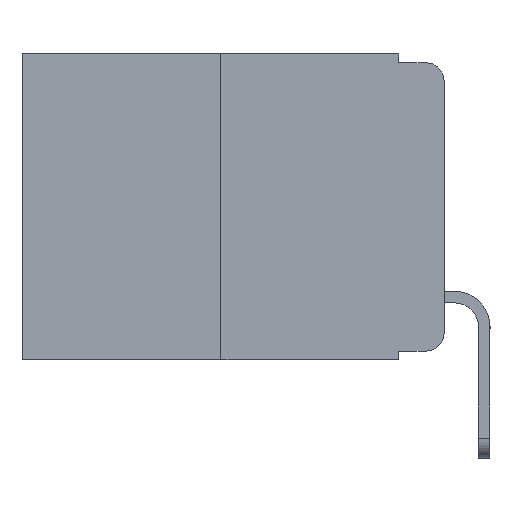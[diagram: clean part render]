
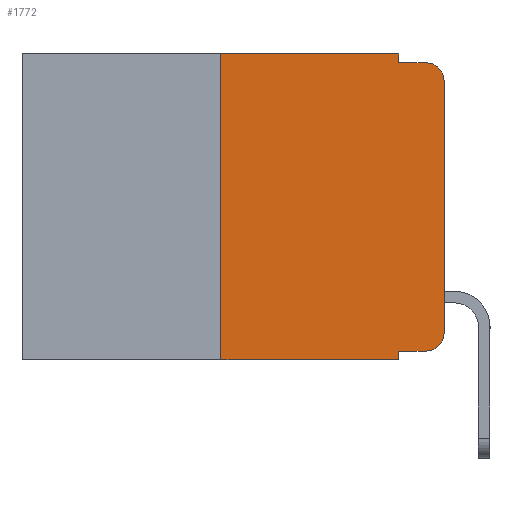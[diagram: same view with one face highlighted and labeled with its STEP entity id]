
A CAD part, left-side view. The second image highlights one B-rep face of the part: STEP entity #1772.
In plain terms, the highlighted planar face has unit normal (-1, 0, 0).
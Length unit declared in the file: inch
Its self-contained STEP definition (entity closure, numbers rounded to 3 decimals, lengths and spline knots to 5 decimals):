
#3 = CARTESIAN_POINT ( 'NONE',  ( 0., 0., -0.03 ) ) ;
#435 = CARTESIAN_POINT ( 'NONE',  ( 0., 0.051, -0.343 ) ) ;
#525 = CIRCLE ( 'NONE', #10193, 0.02 ) ;
#559 = VECTOR ( 'NONE', #13031, 39.37008 ) ;
#737 = PLANE ( 'NONE',  #944 ) ;
#944 = AXIS2_PLACEMENT_3D ( 'NONE', #10278, #2093, #10332 ) ;
#952 = VECTOR ( 'NONE', #11811, 39.37008 ) ;
#982 = CARTESIAN_POINT ( 'NONE',  ( 0., 0., 0. ) ) ;
#1042 = CARTESIAN_POINT ( 'NONE',  ( 0., 0.02, -0.03 ) ) ;
#1159 = DIRECTION ( 'NONE',  ( 0., 0., 1. ) ) ;
#1585 = CARTESIAN_POINT ( 'NONE',  ( 0., 0.25, -0.343 ) ) ;
#1772 = ADVANCED_FACE ( 'NONE', ( #8303 ), #737, .F. ) ;
#2093 = DIRECTION ( 'NONE',  ( 1., 0., 0. ) ) ;
#2400 = DIRECTION ( 'NONE',  ( 0., 0., -1. ) ) ;
#2480 = ORIENTED_EDGE ( 'NONE', *, *, #14146, .F. ) ;
#2523 = CARTESIAN_POINT ( 'NONE',  ( 0., 0.051, 0. ) ) ;
#2577 = CARTESIAN_POINT ( 'NONE',  ( 0., 0.02, -0.313 ) ) ;
#2683 = ORIENTED_EDGE ( 'NONE', *, *, #13733, .T. ) ;
#2843 = VERTEX_POINT ( 'NONE', #435 ) ;
#3191 = VERTEX_POINT ( 'NONE', #13939 ) ;
#3212 = ORIENTED_EDGE ( 'NONE', *, *, #14189, .F. ) ;
#3463 = CARTESIAN_POINT ( 'NONE',  ( 0., 0.051, 0. ) ) ;
#3483 = ORIENTED_EDGE ( 'NONE', *, *, #14217, .T. ) ;
#3598 = ORIENTED_EDGE ( 'NONE', *, *, #13000, .F. ) ;
#3653 = ORIENTED_EDGE ( 'NONE', *, *, #14213, .T. ) ;
#3760 = DIRECTION ( 'NONE',  ( 0., 0., -1. ) ) ;
#3932 = LINE ( 'NONE', #4979, #9795 ) ;
#4014 = VERTEX_POINT ( 'NONE', #11458 ) ;
#4200 = VERTEX_POINT ( 'NONE', #3 ) ;
#4308 = VECTOR ( 'NONE', #14018, 39.37008 ) ;
#4537 = VERTEX_POINT ( 'NONE', #11163 ) ;
#4918 = CARTESIAN_POINT ( 'NONE',  ( 0., 0.051, 0. ) ) ;
#4979 = CARTESIAN_POINT ( 'NONE',  ( 0., 0.051, -0.333 ) ) ;
#5144 = ORIENTED_EDGE ( 'NONE', *, *, #14194, .F. ) ;
#5331 = CARTESIAN_POINT ( 'NONE',  ( 0., 0.051, -0.01 ) ) ;
#5523 = LINE ( 'NONE', #7201, #13784 ) ;
#5744 = VERTEX_POINT ( 'NONE', #11231 ) ;
#6049 = DIRECTION ( 'NONE',  ( 0., 0., 1. ) ) ;
#6200 = DIRECTION ( 'NONE',  ( 0., -1., 0. ) ) ;
#6271 = VERTEX_POINT ( 'NONE', #5331 ) ;
#7156 = LINE ( 'NONE', #2523, #952 ) ;
#7177 = ORIENTED_EDGE ( 'NONE', *, *, #14142, .T. ) ;
#7187 = AXIS2_PLACEMENT_3D ( 'NONE', #1042, #9477, #2400 ) ;
#7201 = CARTESIAN_POINT ( 'NONE',  ( 0., 0.051, -0.01 ) ) ;
#7939 = EDGE_LOOP ( 'NONE', ( #8387, #7177, #2480, #3212, #3598, #5144, #2683, #8847, #3653, #3483 ) ) ;
#8208 = VECTOR ( 'NONE', #6049, 39.37008 ) ;
#8303 = FACE_OUTER_BOUND ( 'NONE', #7939, .T. ) ;
#8347 = DIRECTION ( 'NONE',  ( 0., -1., 0. ) ) ;
#8387 = ORIENTED_EDGE ( 'NONE', *, *, #14138, .T. ) ;
#8847 = ORIENTED_EDGE ( 'NONE', *, *, #14210, .F. ) ;
#9427 = VERTEX_POINT ( 'NONE', #13525 ) ;
#9477 = DIRECTION ( 'NONE',  ( -1., 0., 0. ) ) ;
#9795 = VECTOR ( 'NONE', #6200, 39.37008 ) ;
#9825 = LINE ( 'NONE', #11950, #559 ) ;
#10141 = VECTOR ( 'NONE', #1159, 39.37008 ) ;
#10193 = AXIS2_PLACEMENT_3D ( 'NONE', #2577, #10723, #3760 ) ;
#10278 = CARTESIAN_POINT ( 'NONE',  ( 0., 0.473, 0. ) ) ;
#10332 = DIRECTION ( 'NONE',  ( 0., 0., -1. ) ) ;
#10476 = LINE ( 'NONE', #4918, #14175 ) ;
#10723 = DIRECTION ( 'NONE',  ( -1., 0., 0. ) ) ;
#10747 = VERTEX_POINT ( 'NONE', #3463 ) ;
#11161 = LINE ( 'NONE', #982, #8208 ) ;
#11163 = CARTESIAN_POINT ( 'NONE',  ( 0., 0.02, -0.01 ) ) ;
#11231 = CARTESIAN_POINT ( 'NONE',  ( 0., 0., -0.313 ) ) ;
#11458 = CARTESIAN_POINT ( 'NONE',  ( 0., 0.02, -0.333 ) ) ;
#11525 = CIRCLE ( 'NONE', #7187, 0.02 ) ;
#11759 = DIRECTION ( 'NONE',  ( 0., 0., -1. ) ) ;
#11811 = DIRECTION ( 'NONE',  ( 0., 0., -1. ) ) ;
#11950 = CARTESIAN_POINT ( 'NONE',  ( 0., 0.473, 0. ) ) ;
#12831 = CARTESIAN_POINT ( 'NONE',  ( 0., 0.25, 0. ) ) ;
#12842 = CARTESIAN_POINT ( 'NONE',  ( 0., 0.473, -0.343 ) ) ;
#13000 = EDGE_CURVE ( 'NONE', #9427, #10747, #9825, .T. ) ;
#13031 = DIRECTION ( 'NONE',  ( 0., -1., 0. ) ) ;
#13064 = LINE ( 'NONE', #12842, #4308 ) ;
#13069 = LINE ( 'NONE', #12831, #10141 ) ;
#13444 = VERTEX_POINT ( 'NONE', #1585 ) ;
#13525 = CARTESIAN_POINT ( 'NONE',  ( 0., 0.25, 0. ) ) ;
#13733 = EDGE_CURVE ( 'NONE', #13444, #2843, #13064, .T. ) ;
#13784 = VECTOR ( 'NONE', #8347, 39.37008 ) ;
#13939 = CARTESIAN_POINT ( 'NONE',  ( 0., 0.051, -0.333 ) ) ;
#14018 = DIRECTION ( 'NONE',  ( 0., -1., 0. ) ) ;
#14138 = EDGE_CURVE ( 'NONE', #5744, #4200, #11161, .T. ) ;
#14142 = EDGE_CURVE ( 'NONE', #4200, #4537, #11525, .T. ) ;
#14146 = EDGE_CURVE ( 'NONE', #6271, #4537, #5523, .T. ) ;
#14175 = VECTOR ( 'NONE', #11759, 39.37008 ) ;
#14189 = EDGE_CURVE ( 'NONE', #10747, #6271, #10476, .T. ) ;
#14194 = EDGE_CURVE ( 'NONE', #13444, #9427, #13069, .T. ) ;
#14210 = EDGE_CURVE ( 'NONE', #3191, #2843, #7156, .T. ) ;
#14213 = EDGE_CURVE ( 'NONE', #3191, #4014, #3932, .T. ) ;
#14217 = EDGE_CURVE ( 'NONE', #4014, #5744, #525, .T. ) ;
